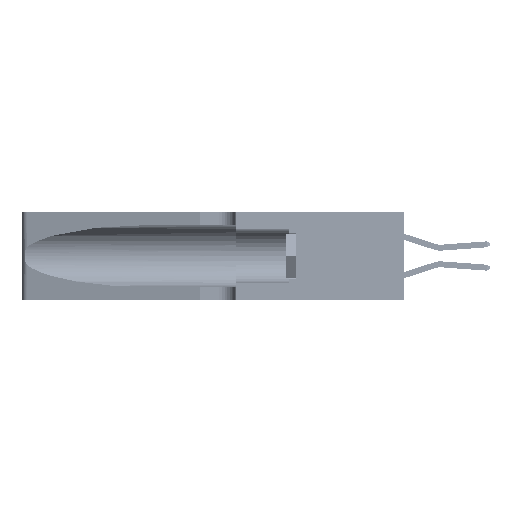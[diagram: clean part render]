
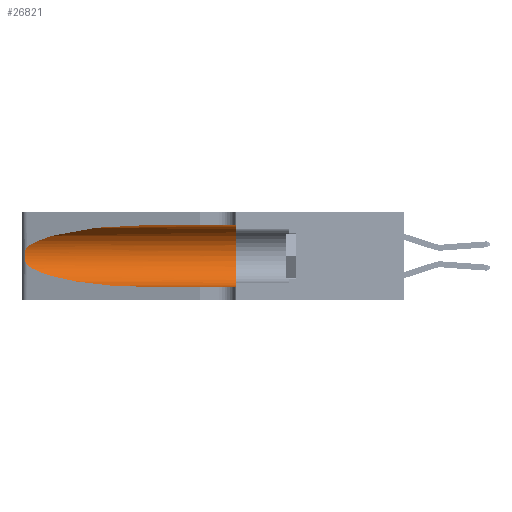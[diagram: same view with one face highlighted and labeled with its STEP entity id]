
A CAD part, left-side view. The second image highlights one B-rep face of the part: STEP entity #26821.
In plain terms, the highlighted cylindrical face has radius 3.308 mm (diameter 6.617 mm), a partial arc.
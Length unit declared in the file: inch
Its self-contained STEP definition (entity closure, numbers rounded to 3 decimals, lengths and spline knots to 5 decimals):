
#637 = CARTESIAN_POINT ( 'NONE',  ( 0.25555, 1.22994, 0.2215 ) ) ;
#1571 = ORIENTED_EDGE ( 'NONE', *, *, #4909, .T. ) ;
#1829 = CARTESIAN_POINT ( 'NONE',  ( 0.1305, 0.72297, 0.05475 ) ) ;
#2112 = CIRCLE ( 'NONE', #5839, 0.13025 ) ;
#3764 = CARTESIAN_POINT ( 'NONE',  ( 0.1305, 1.61858, 0.31525 ) ) ;
#4191 = CARTESIAN_POINT ( 'NONE',  ( 0.25787, 1.23484, 0.2124 ) ) ;
#4243 = ORIENTED_EDGE ( 'NONE', *, *, #6245, .F. ) ;
#4909 = EDGE_CURVE ( 'NONE', #23870, #21379, #32845, .T. ) ;
#5839 = AXIS2_PLACEMENT_3D ( 'NONE', #11710, #40209, #10762 ) ;
#6245 = EDGE_CURVE ( 'NONE', #35434, #25748, #2112, .T. ) ;
#7930 = CARTESIAN_POINT ( 'NONE',  ( 0.25789, 1.23486, 0.15765 ) ) ;
#7979 = DIRECTION ( 'NONE',  ( 0., -1., 0. ) ) ;
#8265 = EDGE_LOOP ( 'NONE', ( #35045, #1571, #9376, #25929, #4243, #10116 ) ) ;
#9376 = ORIENTED_EDGE ( 'NONE', *, *, #23909, .T. ) ;
#10116 = ORIENTED_EDGE ( 'NONE', *, *, #40642, .F. ) ;
#10762 = DIRECTION ( 'NONE',  ( 0., 0., 1. ) ) ;
#11710 = CARTESIAN_POINT ( 'NONE',  ( 0.1305, 0.35, 0.185 ) ) ;
#11755 = CARTESIAN_POINT ( 'NONE',  ( 0.25487, 1.22718, 0.22369 ) ) ;
#12379 = VERTEX_POINT ( 'NONE', #38776 ) ;
#13605 = CARTESIAN_POINT ( 'NONE',  ( 0.1305, 0.72297, 0.31525 ) ) ;
#14979 = CARTESIAN_POINT ( 'NONE',  ( 0.25639, 1.23184, 0.21858 ) ) ;
#15479 = VECTOR ( 'NONE', #30223, 39.37008 ) ;
#15709 =( BOUNDED_CURVE ( )  B_SPLINE_CURVE ( 3, ( #13605, #21332, #24908, #28479 ),
 .UNSPECIFIED., .F., .F. ) 
 B_SPLINE_CURVE_WITH_KNOTS ( ( 4, 4 ),
 ( 1.5708, 2.84003 ),
 .UNSPECIFIED. ) 
 CURVE ( )  GEOMETRIC_REPRESENTATION_ITEM ( )  RATIONAL_B_SPLINE_CURVE ( ( 1., 0.87, 0.87, 1. ) ) 
 REPRESENTATION_ITEM ( '' )  );
#16478 = CARTESIAN_POINT ( 'NONE',  ( 0.18966, 0.96281, 0.05475 ) ) ;
#16649 = LINE ( 'NONE', #3764, #15479 ) ;
#18839 = CARTESIAN_POINT ( 'NONE',  ( 0.26017, 1.23833, 0.17102 ) ) ;
#18893 = CARTESIAN_POINT ( 'NONE',  ( 0.1305, 1.61858, 0.185 ) ) ;
#19164 = CARTESIAN_POINT ( 'NONE',  ( 0.25854, 1.2359, 0.20912 ) ) ;
#20755 = LINE ( 'NONE', #21282, #23082 ) ;
#21282 = CARTESIAN_POINT ( 'NONE',  ( 0.1305, 1.61858, 0.05475 ) ) ;
#21332 = CARTESIAN_POINT ( 'NONE',  ( 0.18966, 0.96281, 0.31525 ) ) ;
#21379 = VERTEX_POINT ( 'NONE', #28620 ) ;
#22569 = CARTESIAN_POINT ( 'NONE',  ( 0.25856, 1.23593, 0.16098 ) ) ;
#22879 = CARTESIAN_POINT ( 'NONE',  ( 0.25487, 1.22718, 0.14631 ) ) ;
#23082 = VECTOR ( 'NONE', #28426, 39.37008 ) ;
#23870 = VERTEX_POINT ( 'NONE', #27782 ) ;
#23909 = EDGE_CURVE ( 'NONE', #21379, #12379, #41994, .T. ) ;
#24908 = CARTESIAN_POINT ( 'NONE',  ( 0.2373, 1.15595, 0.28018 ) ) ;
#25748 = VERTEX_POINT ( 'NONE', #37821 ) ;
#25929 = ORIENTED_EDGE ( 'NONE', *, *, #40147, .T. ) ;
#26123 = CARTESIAN_POINT ( 'NONE',  ( 0.25555, 1.22993, 0.14849 ) ) ;
#26821 = ADVANCED_FACE ( 'NONE', ( #34384 ), #27475, .F. ) ;
#27475 = CYLINDRICAL_SURFACE ( 'NONE', #29058, 0.13025 ) ;
#27782 = CARTESIAN_POINT ( 'NONE',  ( 0.25487, 1.22718, 0.22369 ) ) ;
#28426 = DIRECTION ( 'NONE',  ( 0., -1., 0. ) ) ;
#28479 = CARTESIAN_POINT ( 'NONE',  ( 0.25487, 1.22718, 0.22369 ) ) ;
#28620 = CARTESIAN_POINT ( 'NONE',  ( 0.25487, 1.22718, 0.14631 ) ) ;
#29058 = AXIS2_PLACEMENT_3D ( 'NONE', #18893, #7979, #44489 ) ;
#29671 = CARTESIAN_POINT ( 'NONE',  ( 0.26018, 1.23835, 0.19895 ) ) ;
#30001 = CARTESIAN_POINT ( 'NONE',  ( 0.26075, 1.23896, 0.178 ) ) ;
#30223 = DIRECTION ( 'NONE',  ( 0., -1., 0. ) ) ;
#32628 = EDGE_CURVE ( 'NONE', #46532, #23870, #15709, .T. ) ;
#32845 = B_SPLINE_CURVE_WITH_KNOTS ( 'NONE', 3,
 ( #11755, #637, #14979, #4191, #19164, #29671, #44923, #30001, #18839, #22569, #7930, #37225, #26123, #22879 ),
 .UNSPECIFIED., .F., .F.,
 ( 4, 2, 2, 2, 2, 2, 4 ),
 ( 0., 0.00027, 0.00053, 0.00107, 0.0016, 0.00187, 0.00214 ),
 .UNSPECIFIED. ) ;
#34384 = FACE_OUTER_BOUND ( 'NONE', #8265, .T. ) ;
#34578 = CARTESIAN_POINT ( 'NONE',  ( 0.1305, 0.35, 0.31525 ) ) ;
#35045 = ORIENTED_EDGE ( 'NONE', *, *, #32628, .T. ) ;
#35434 = VERTEX_POINT ( 'NONE', #34578 ) ;
#37225 = CARTESIAN_POINT ( 'NONE',  ( 0.25639, 1.23186, 0.15144 ) ) ;
#37821 = CARTESIAN_POINT ( 'NONE',  ( 0.1305, 0.35, 0.05475 ) ) ;
#38520 = CARTESIAN_POINT ( 'NONE',  ( 0.25487, 1.22718, 0.14631 ) ) ;
#38776 = CARTESIAN_POINT ( 'NONE',  ( 0.1305, 0.72297, 0.05475 ) ) ;
#40082 = CARTESIAN_POINT ( 'NONE',  ( 0.1305, 0.72297, 0.31525 ) ) ;
#40147 = EDGE_CURVE ( 'NONE', #12379, #25748, #20755, .T. ) ;
#40209 = DIRECTION ( 'NONE',  ( 0., 1., 0. ) ) ;
#40642 = EDGE_CURVE ( 'NONE', #46532, #35434, #16649, .T. ) ;
#41994 =( BOUNDED_CURVE ( )  B_SPLINE_CURVE ( 3, ( #38520, #46239, #16478, #1829 ),
 .UNSPECIFIED., .F., .F. ) 
 B_SPLINE_CURVE_WITH_KNOTS ( ( 4, 4 ),
 ( 3.44316, 4.71239 ),
 .UNSPECIFIED. ) 
 CURVE ( )  GEOMETRIC_REPRESENTATION_ITEM ( )  RATIONAL_B_SPLINE_CURVE ( ( 1., 0.87, 0.87, 1. ) ) 
 REPRESENTATION_ITEM ( '' )  );
#44489 = DIRECTION ( 'NONE',  ( 0., 0., -1. ) ) ;
#44923 = CARTESIAN_POINT ( 'NONE',  ( 0.26075, 1.23896, 0.19203 ) ) ;
#46239 = CARTESIAN_POINT ( 'NONE',  ( 0.2373, 1.15595, 0.08982 ) ) ;
#46532 = VERTEX_POINT ( 'NONE', #40082 ) ;
